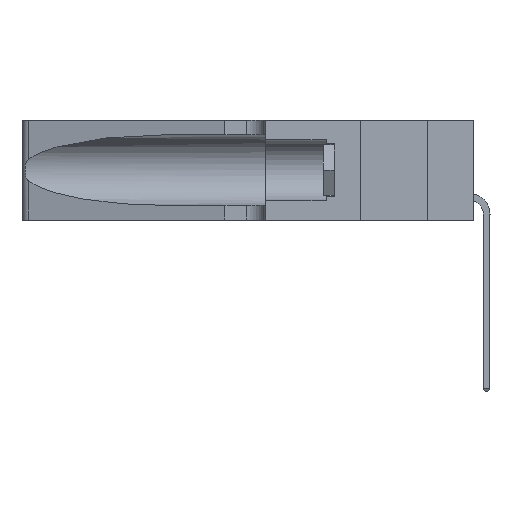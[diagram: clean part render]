
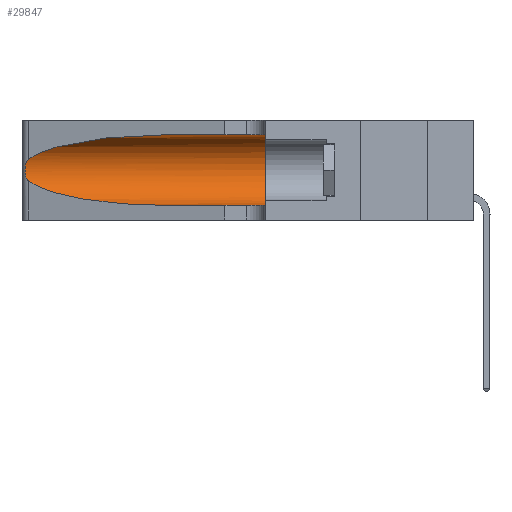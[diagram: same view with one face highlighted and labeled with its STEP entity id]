
A CAD part, left-side view. The second image highlights one B-rep face of the part: STEP entity #29847.
In plain terms, the highlighted cylindrical face has radius 3.308 mm (diameter 6.617 mm), a partial arc.
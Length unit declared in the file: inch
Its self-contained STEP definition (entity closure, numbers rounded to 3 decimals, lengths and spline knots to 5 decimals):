
#45 = CARTESIAN_POINT ( 'NONE',  ( 0.1305, 1.61858, 0.05475 ) ) ;
#173 = CARTESIAN_POINT ( 'NONE',  ( 0.25856, 1.23593, 0.16098 ) ) ;
#1215 = CARTESIAN_POINT ( 'NONE',  ( 0.1305, 0.35, 0.31525 ) ) ;
#2872 = CARTESIAN_POINT ( 'NONE',  ( 0.1305, 0.35, 0.185 ) ) ;
#3888 = EDGE_CURVE ( 'NONE', #10705, #5602, #25414, .T. ) ;
#4268 = CARTESIAN_POINT ( 'NONE',  ( 0.26018, 1.23835, 0.19895 ) ) ;
#4644 = EDGE_CURVE ( 'NONE', #19974, #18149, #12060, .T. ) ;
#5602 = VERTEX_POINT ( 'NONE', #1215 ) ;
#5904 = VERTEX_POINT ( 'NONE', #22607 ) ;
#6070 =( BOUNDED_CURVE ( )  B_SPLINE_CURVE ( 3, ( #26945, #9615, #11614, #20269 ),
 .UNSPECIFIED., .F., .T. ) 
 B_SPLINE_CURVE_WITH_KNOTS ( ( 4, 4 ),
 ( 3.44316, 4.71239 ),
 .UNSPECIFIED. ) 
 CURVE ( )  GEOMETRIC_REPRESENTATION_ITEM ( )  RATIONAL_B_SPLINE_CURVE ( ( 1., 0.87, 0.87, 1. ) ) 
 REPRESENTATION_ITEM ( '' )  );
#6405 = ORIENTED_EDGE ( 'NONE', *, *, #4644, .T. ) ;
#6757 = CARTESIAN_POINT ( 'NONE',  ( 0.1305, 1.61858, 0.31525 ) ) ;
#7107 = VECTOR ( 'NONE', #17082, 39.37008 ) ;
#7147 = CARTESIAN_POINT ( 'NONE',  ( 0.26075, 1.23896, 0.19203 ) ) ;
#7431 = CARTESIAN_POINT ( 'NONE',  ( 0.25639, 1.23186, 0.15144 ) ) ;
#8774 = EDGE_CURVE ( 'NONE', #5904, #19974, #6070, .T. ) ;
#9355 = CARTESIAN_POINT ( 'NONE',  ( 0.1305, 0.35, 0.05475 ) ) ;
#9531 = CARTESIAN_POINT ( 'NONE',  ( 0.1305, 1.61858, 0.185 ) ) ;
#9615 = CARTESIAN_POINT ( 'NONE',  ( 0.2373, 1.15595, 0.08982 ) ) ;
#9831 = DIRECTION ( 'NONE',  ( 0., 0., -1. ) ) ;
#10705 = VERTEX_POINT ( 'NONE', #13693 ) ;
#10711 = CARTESIAN_POINT ( 'NONE',  ( 0.25487, 1.22718, 0.22369 ) ) ;
#10822 = CIRCLE ( 'NONE', #22910, 0.13025 ) ;
#11614 = CARTESIAN_POINT ( 'NONE',  ( 0.18966, 0.96281, 0.05475 ) ) ;
#12060 = LINE ( 'NONE', #45, #7107 ) ;
#12132 = EDGE_CURVE ( 'NONE', #27519, #5904, #17941, .T. ) ;
#12725 = CARTESIAN_POINT ( 'NONE',  ( 0.1305, 0.72297, 0.05475 ) ) ;
#13165 = FACE_OUTER_BOUND ( 'NONE', #24287, .T. ) ;
#13693 = CARTESIAN_POINT ( 'NONE',  ( 0.1305, 0.72297, 0.31525 ) ) ;
#13698 = EDGE_CURVE ( 'NONE', #10705, #27519, #20291, .T. ) ;
#14193 = CARTESIAN_POINT ( 'NONE',  ( 0.25487, 1.22718, 0.22369 ) ) ;
#14444 = DIRECTION ( 'NONE',  ( 0., -1., 0. ) ) ;
#15423 = ORIENTED_EDGE ( 'NONE', *, *, #12132, .T. ) ;
#15727 = CARTESIAN_POINT ( 'NONE',  ( 0.2373, 1.15595, 0.28018 ) ) ;
#16248 = AXIS2_PLACEMENT_3D ( 'NONE', #9531, #14444, #9831 ) ;
#16924 = CARTESIAN_POINT ( 'NONE',  ( 0.26017, 1.23833, 0.17102 ) ) ;
#17082 = DIRECTION ( 'NONE',  ( 0., -1., 0. ) ) ;
#17243 = DIRECTION ( 'NONE',  ( 0., 0., 1. ) ) ;
#17941 = B_SPLINE_CURVE_WITH_KNOTS ( 'NONE', 3,
 ( #14193, #28530, #28849, #18870, #31182, #4268, #7147, #22111, #16924, #173, #26788, #7431, #24437, #21801 ),
 .UNSPECIFIED., .F., .F.,
 ( 4, 2, 2, 2, 2, 2, 4 ),
 ( 0., 0.00027, 0.00053, 0.00107, 0.0016, 0.00187, 0.00214 ),
 .UNSPECIFIED. ) ;
#18043 = CARTESIAN_POINT ( 'NONE',  ( 0.1305, 0.72297, 0.31525 ) ) ;
#18149 = VERTEX_POINT ( 'NONE', #9355 ) ;
#18497 = CYLINDRICAL_SURFACE ( 'NONE', #16248, 0.13025 ) ;
#18870 = CARTESIAN_POINT ( 'NONE',  ( 0.25787, 1.23484, 0.2124 ) ) ;
#19915 = DIRECTION ( 'NONE',  ( 0., 1., 0. ) ) ;
#19974 = VERTEX_POINT ( 'NONE', #12725 ) ;
#20269 = CARTESIAN_POINT ( 'NONE',  ( 0.1305, 0.72297, 0.05475 ) ) ;
#20291 =( BOUNDED_CURVE ( )  B_SPLINE_CURVE ( 3, ( #18043, #25261, #15727, #10711 ),
 .UNSPECIFIED., .F., .F. ) 
 B_SPLINE_CURVE_WITH_KNOTS ( ( 4, 4 ),
 ( 1.5708, 2.84003 ),
 .UNSPECIFIED. ) 
 CURVE ( )  GEOMETRIC_REPRESENTATION_ITEM ( )  RATIONAL_B_SPLINE_CURVE ( ( 1., 0.87, 0.87, 1. ) ) 
 REPRESENTATION_ITEM ( '' )  );
#21542 = ORIENTED_EDGE ( 'NONE', *, *, #3888, .F. ) ;
#21801 = CARTESIAN_POINT ( 'NONE',  ( 0.25487, 1.22718, 0.14631 ) ) ;
#22111 = CARTESIAN_POINT ( 'NONE',  ( 0.26075, 1.23896, 0.178 ) ) ;
#22607 = CARTESIAN_POINT ( 'NONE',  ( 0.25487, 1.22718, 0.14631 ) ) ;
#22910 = AXIS2_PLACEMENT_3D ( 'NONE', #2872, #19915, #17243 ) ;
#24287 = EDGE_LOOP ( 'NONE', ( #28882, #15423, #29762, #6405, #28510, #21542 ) ) ;
#24437 = CARTESIAN_POINT ( 'NONE',  ( 0.25555, 1.22993, 0.14849 ) ) ;
#24639 = VECTOR ( 'NONE', #28878, 39.37008 ) ;
#25261 = CARTESIAN_POINT ( 'NONE',  ( 0.18966, 0.96281, 0.31525 ) ) ;
#25414 = LINE ( 'NONE', #6757, #24639 ) ;
#26788 = CARTESIAN_POINT ( 'NONE',  ( 0.25789, 1.23486, 0.15765 ) ) ;
#26945 = CARTESIAN_POINT ( 'NONE',  ( 0.25487, 1.22718, 0.14631 ) ) ;
#27519 = VERTEX_POINT ( 'NONE', #29529 ) ;
#28510 = ORIENTED_EDGE ( 'NONE', *, *, #28738, .F. ) ;
#28530 = CARTESIAN_POINT ( 'NONE',  ( 0.25555, 1.22994, 0.2215 ) ) ;
#28738 = EDGE_CURVE ( 'NONE', #5602, #18149, #10822, .T. ) ;
#28849 = CARTESIAN_POINT ( 'NONE',  ( 0.25639, 1.23184, 0.21858 ) ) ;
#28878 = DIRECTION ( 'NONE',  ( 0., -1., 0. ) ) ;
#28882 = ORIENTED_EDGE ( 'NONE', *, *, #13698, .T. ) ;
#29529 = CARTESIAN_POINT ( 'NONE',  ( 0.25487, 1.22718, 0.22369 ) ) ;
#29762 = ORIENTED_EDGE ( 'NONE', *, *, #8774, .T. ) ;
#29847 = ADVANCED_FACE ( 'NONE', ( #13165 ), #18497, .F. ) ;
#31182 = CARTESIAN_POINT ( 'NONE',  ( 0.25854, 1.2359, 0.20912 ) ) ;
